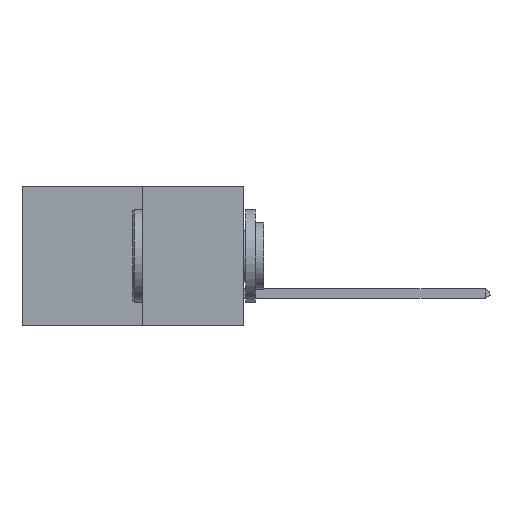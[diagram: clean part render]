
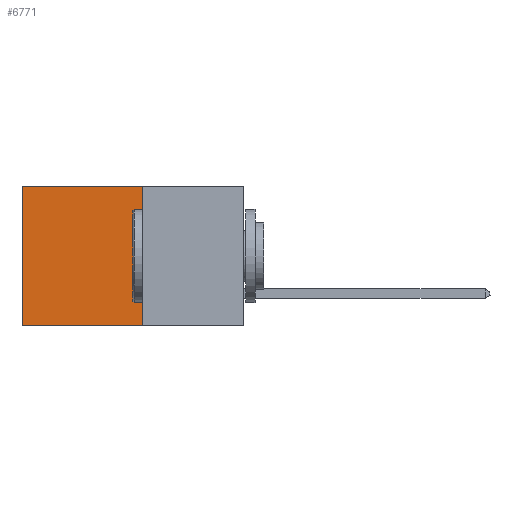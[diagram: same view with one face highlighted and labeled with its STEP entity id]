
A CAD part, left-side view. The second image highlights one B-rep face of the part: STEP entity #6771.
In plain terms, the highlighted planar face has unit normal (-1, 0, 0).
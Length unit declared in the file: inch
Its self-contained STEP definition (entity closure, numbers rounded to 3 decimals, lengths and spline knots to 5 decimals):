
#1415 = AXIS2_PLACEMENT_3D ( 'NONE', #4002, #3951, #3925 ) ;
#1437 = DIRECTION ( 'NONE',  ( 0., 0., -1. ) ) ;
#1481 = LINE ( 'NONE', #9341, #15744 ) ;
#1566 = CARTESIAN_POINT ( 'NONE',  ( 0.277, 0.27, -0.37 ) ) ;
#2647 = CARTESIAN_POINT ( 'NONE',  ( 0.277, 0.59, -0.37 ) ) ;
#2963 = CARTESIAN_POINT ( 'NONE',  ( 0.277, 0.59, -0.37 ) ) ;
#3338 = ORIENTED_EDGE ( 'NONE', *, *, #17570, .F. ) ;
#3383 = CARTESIAN_POINT ( 'NONE',  ( 0.277, 0.27, 0. ) ) ;
#3925 = DIRECTION ( 'NONE',  ( 0., 0., -1. ) ) ;
#3951 = DIRECTION ( 'NONE',  ( 1., 0., 0. ) ) ;
#4002 = CARTESIAN_POINT ( 'NONE',  ( 0.277, 0.27, -0.37 ) ) ;
#4154 = PLANE ( 'NONE',  #1415 ) ;
#4668 = EDGE_LOOP ( 'NONE', ( #12790, #3338, #18287, #13761 ) ) ;
#5128 = EDGE_CURVE ( 'NONE', #5697, #14364, #11260, .T. ) ;
#5697 = VERTEX_POINT ( 'NONE', #22852 ) ;
#5949 = VECTOR ( 'NONE', #1437, 39.37008 ) ;
#6520 = DIRECTION ( 'NONE',  ( 0., 0., -1. ) ) ;
#6771 = ADVANCED_FACE ( 'NONE', ( #6970 ), #4154, .F. ) ;
#6831 = VERTEX_POINT ( 'NONE', #2647 ) ;
#6970 = FACE_OUTER_BOUND ( 'NONE', #4668, .T. ) ;
#7373 = LINE ( 'NONE', #3383, #12130 ) ;
#9341 = CARTESIAN_POINT ( 'NONE',  ( 0.277, 0.27, -0.37 ) ) ;
#10913 = CARTESIAN_POINT ( 'NONE',  ( 0.277, 0.59, 0. ) ) ;
#11260 = LINE ( 'NONE', #1566, #5949 ) ;
#12130 = VECTOR ( 'NONE', #15890, 39.37008 ) ;
#12790 = ORIENTED_EDGE ( 'NONE', *, *, #15318, .T. ) ;
#13761 = ORIENTED_EDGE ( 'NONE', *, *, #16664, .T. ) ;
#14364 = VERTEX_POINT ( 'NONE', #20779 ) ;
#15318 = EDGE_CURVE ( 'NONE', #19452, #6831, #18075, .T. ) ;
#15586 = VECTOR ( 'NONE', #6520, 39.37008 ) ;
#15744 = VECTOR ( 'NONE', #19980, 39.37008 ) ;
#15890 = DIRECTION ( 'NONE',  ( 0., 1., 0. ) ) ;
#16664 = EDGE_CURVE ( 'NONE', #5697, #19452, #7373, .T. ) ;
#17570 = EDGE_CURVE ( 'NONE', #14364, #6831, #1481, .T. ) ;
#18075 = LINE ( 'NONE', #2963, #15586 ) ;
#18287 = ORIENTED_EDGE ( 'NONE', *, *, #5128, .F. ) ;
#19452 = VERTEX_POINT ( 'NONE', #10913 ) ;
#19980 = DIRECTION ( 'NONE',  ( 0., 1., 0. ) ) ;
#20779 = CARTESIAN_POINT ( 'NONE',  ( 0.277, 0.27, -0.37 ) ) ;
#22852 = CARTESIAN_POINT ( 'NONE',  ( 0.277, 0.27, 0. ) ) ;
